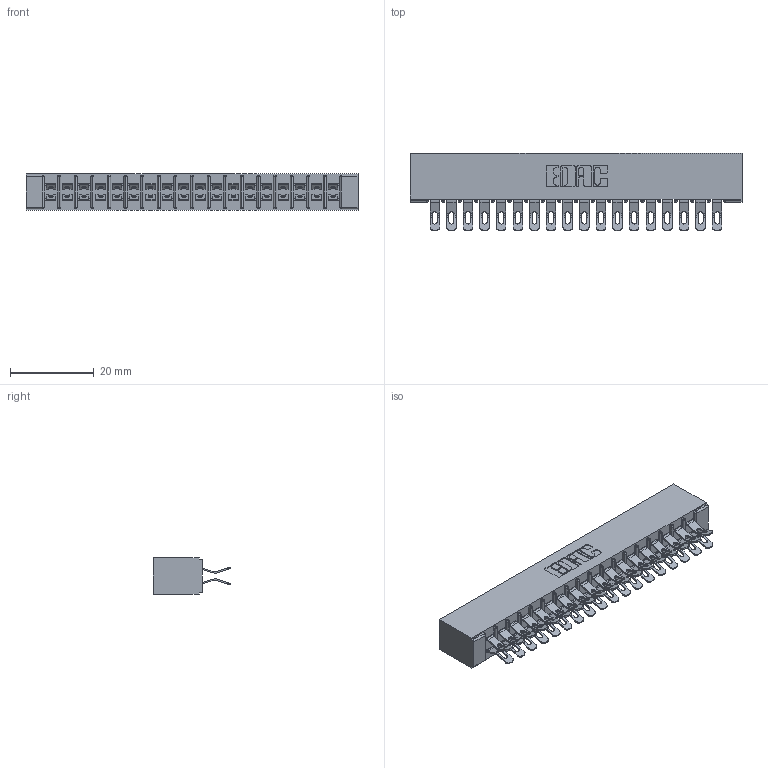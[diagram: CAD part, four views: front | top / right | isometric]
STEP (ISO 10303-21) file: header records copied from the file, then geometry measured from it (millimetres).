
FILE_DESCRIPTION (( 'STEP AP203' ), '1' );
FILE_NAME ('355-036-555-501.STEP', '2019-09-11T09:50:35', ( '' ), ( '' ), 'SwSTEP 2.0', 'SolidWorks 2016', '' );
FILE_SCHEMA (( 'CONFIG_CONTROL_DESIGN' ));
Length unit declared in the file: inch
Products named in the file (3): 305-290-001_555; 355-036-555-501; 305 Part_No Mounting
Assembly tree (37 placements, depth 2):
  355-036-555-501
    305 Part_No Mounting
    305-290-001_555  x36
Bounding box: 79.2 x 18.41 x 8.71 mm (x, y, z)
Volume: 5016.4 mm3; surface area: 10980.8 mm2
Topology: 37 solids, 37 shells, 2484 faces, 7402 edges, 4836 vertices
Faces by surface type: plane 1216, cylinder 1196, sphere 72
Entity records: 22757 total; most frequent: CARTESIAN_POINT 3782, ORIENTED_EDGE 3740, DIRECTION 3670, EDGE_CURVE 1870, LINE 1470, VECTOR 1470, VERTEX_POINT 1196, AXIS2_PLACEMENT_3D 1100
